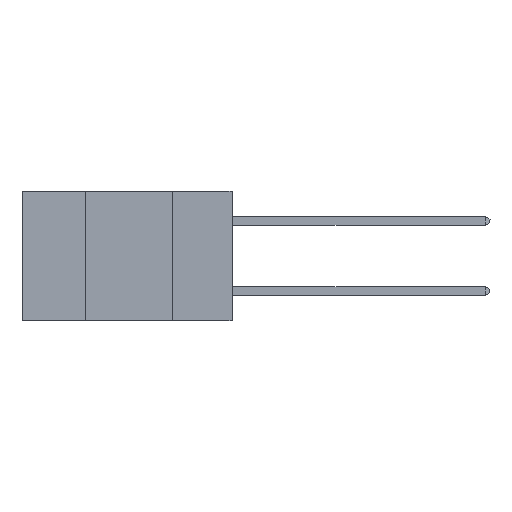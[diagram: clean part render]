
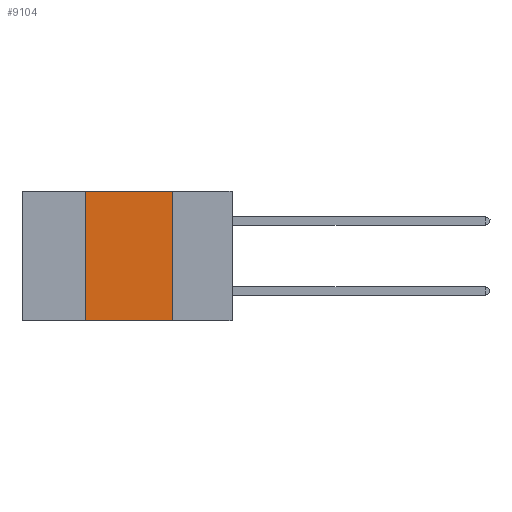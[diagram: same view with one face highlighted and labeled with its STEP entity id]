
A CAD part, left-side view. The second image highlights one B-rep face of the part: STEP entity #9104.
In plain terms, the highlighted planar face has unit normal (-1, 0, 0).
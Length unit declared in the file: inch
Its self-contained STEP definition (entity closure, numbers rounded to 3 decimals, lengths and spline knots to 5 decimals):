
#405 = LINE ( 'NONE', #25461, #21241 ) ;
#757 = DIRECTION ( 'NONE',  ( 0., -1., 0. ) ) ;
#4004 = EDGE_CURVE ( 'NONE', #34768, #35442, #20803, .T. ) ;
#5299 = CARTESIAN_POINT ( 'NONE',  ( 0., 0.17, 0. ) ) ;
#7036 = CARTESIAN_POINT ( 'NONE',  ( 0., 0.42, 0. ) ) ;
#8657 = DIRECTION ( 'NONE',  ( 1., 0., 0. ) ) ;
#9104 = ADVANCED_FACE ( 'NONE', ( #17041 ), #24585, .F. ) ;
#9309 = DIRECTION ( 'NONE',  ( 0., -1., 0. ) ) ;
#13102 = ORIENTED_EDGE ( 'NONE', *, *, #17118, .F. ) ;
#14339 = EDGE_CURVE ( 'NONE', #28984, #37844, #21866, .T. ) ;
#16727 = CARTESIAN_POINT ( 'NONE',  ( 0., 0.42, -0.37 ) ) ;
#17041 = FACE_OUTER_BOUND ( 'NONE', #30619, .T. ) ;
#17118 = EDGE_CURVE ( 'NONE', #37844, #34768, #405, .T. ) ;
#19792 = DIRECTION ( 'NONE',  ( 0., 0., -1. ) ) ;
#20705 = ORIENTED_EDGE ( 'NONE', *, *, #14339, .F. ) ;
#20803 = LINE ( 'NONE', #37791, #33756 ) ;
#21241 = VECTOR ( 'NONE', #757, 39.37008 ) ;
#21394 = CARTESIAN_POINT ( 'NONE',  ( 0., 0.6, 0. ) ) ;
#21866 = LINE ( 'NONE', #7036, #36847 ) ;
#23948 = VECTOR ( 'NONE', #9309, 39.37008 ) ;
#24181 = EDGE_CURVE ( 'NONE', #28984, #35442, #32169, .T. ) ;
#24585 = PLANE ( 'NONE',  #24597 ) ;
#24597 = AXIS2_PLACEMENT_3D ( 'NONE', #21394, #8657, #33501 ) ;
#25137 = ORIENTED_EDGE ( 'NONE', *, *, #4004, .F. ) ;
#25461 = CARTESIAN_POINT ( 'NONE',  ( 0., 0.6, 0. ) ) ;
#25779 = CARTESIAN_POINT ( 'NONE',  ( 0., 0.17, -0.37 ) ) ;
#28984 = VERTEX_POINT ( 'NONE', #16727 ) ;
#30619 = EDGE_LOOP ( 'NONE', ( #25137, #13102, #20705, #35378 ) ) ;
#32169 = LINE ( 'NONE', #38533, #23948 ) ;
#33501 = DIRECTION ( 'NONE',  ( 0., 0., -1. ) ) ;
#33756 = VECTOR ( 'NONE', #19792, 39.37008 ) ;
#34400 = DIRECTION ( 'NONE',  ( 0., 0., 1. ) ) ;
#34768 = VERTEX_POINT ( 'NONE', #5299 ) ;
#35378 = ORIENTED_EDGE ( 'NONE', *, *, #24181, .T. ) ;
#35442 = VERTEX_POINT ( 'NONE', #25779 ) ;
#36847 = VECTOR ( 'NONE', #34400, 39.37008 ) ;
#37336 = CARTESIAN_POINT ( 'NONE',  ( 0., 0.42, 0. ) ) ;
#37791 = CARTESIAN_POINT ( 'NONE',  ( 0., 0.17, 0. ) ) ;
#37844 = VERTEX_POINT ( 'NONE', #37336 ) ;
#38533 = CARTESIAN_POINT ( 'NONE',  ( 0., 0.6, -0.37 ) ) ;
